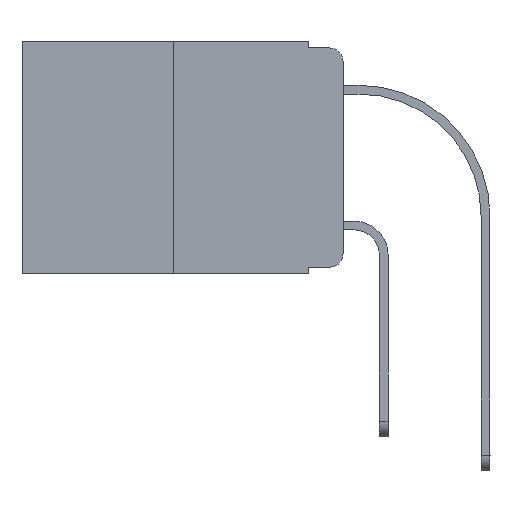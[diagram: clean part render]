
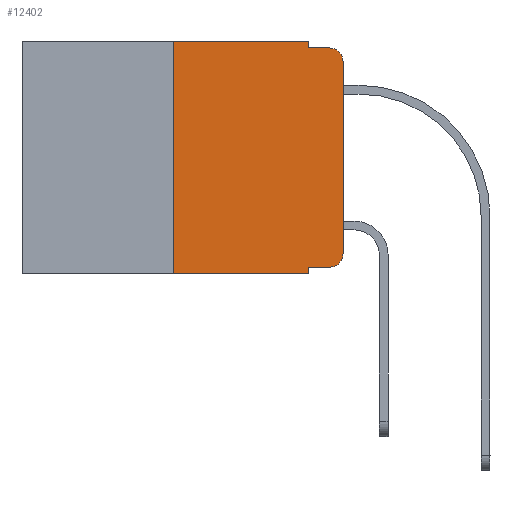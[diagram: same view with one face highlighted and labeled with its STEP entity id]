
A CAD part, left-side view. The second image highlights one B-rep face of the part: STEP entity #12402.
In plain terms, the highlighted planar face has unit normal (-1, 0, 0).
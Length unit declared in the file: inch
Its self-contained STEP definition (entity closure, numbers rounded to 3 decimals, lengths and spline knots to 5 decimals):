
#48 = CARTESIAN_POINT ( 'NONE',  ( 0., 0., -0.03 ) ) ;
#959 = CARTESIAN_POINT ( 'NONE',  ( 0., 0., 0. ) ) ;
#1026 = EDGE_CURVE ( 'NONE', #12357, #7977, #12486, .T. ) ;
#1219 = CARTESIAN_POINT ( 'NONE',  ( 0., 0.473, 0. ) ) ;
#1285 = ORIENTED_EDGE ( 'NONE', *, *, #20012, .F. ) ;
#1403 = DIRECTION ( 'NONE',  ( 0., -1., 0. ) ) ;
#2087 = CARTESIAN_POINT ( 'NONE',  ( 0., 0.051, 0. ) ) ;
#2621 = CARTESIAN_POINT ( 'NONE',  ( 0., 0.051, 0. ) ) ;
#2697 = ORIENTED_EDGE ( 'NONE', *, *, #5243, .F. ) ;
#3816 = ORIENTED_EDGE ( 'NONE', *, *, #8932, .T. ) ;
#4022 = DIRECTION ( 'NONE',  ( -1., 0., 0. ) ) ;
#4285 = CARTESIAN_POINT ( 'NONE',  ( 0., 0.051, -0.01 ) ) ;
#4560 = VERTEX_POINT ( 'NONE', #48 ) ;
#4965 = CIRCLE ( 'NONE', #16002, 0.02 ) ;
#5157 = EDGE_CURVE ( 'NONE', #23878, #4560, #9009, .T. ) ;
#5243 = EDGE_CURVE ( 'NONE', #7963, #17933, #9674, .T. ) ;
#5247 = DIRECTION ( 'NONE',  ( 0., 0., 1. ) ) ;
#5505 = EDGE_LOOP ( 'NONE', ( #9695, #7237, #6449, #23156, #2697, #14933, #5924, #1285, #17337, #3816 ) ) ;
#5670 = AXIS2_PLACEMENT_3D ( 'NONE', #8058, #4022, #8195 ) ;
#5687 = VECTOR ( 'NONE', #26960, 39.37008 ) ;
#5924 = ORIENTED_EDGE ( 'NONE', *, *, #17755, .T. ) ;
#6449 = ORIENTED_EDGE ( 'NONE', *, *, #12979, .F. ) ;
#7237 = ORIENTED_EDGE ( 'NONE', *, *, #14172, .T. ) ;
#7654 = VECTOR ( 'NONE', #1403, 39.37008 ) ;
#7759 = CARTESIAN_POINT ( 'NONE',  ( 0., 0.051, -0.343 ) ) ;
#7963 = VERTEX_POINT ( 'NONE', #9833 ) ;
#7977 = VERTEX_POINT ( 'NONE', #13708 ) ;
#8058 = CARTESIAN_POINT ( 'NONE',  ( 0., 0.02, -0.03 ) ) ;
#8102 = DIRECTION ( 'NONE',  ( 0., 0., -1. ) ) ;
#8195 = DIRECTION ( 'NONE',  ( 0., 0., -1. ) ) ;
#8223 = CARTESIAN_POINT ( 'NONE',  ( 0., 0.473, 0. ) ) ;
#8375 = VECTOR ( 'NONE', #5247, 39.37008 ) ;
#8598 = DIRECTION ( 'NONE',  ( 0., -1., 0. ) ) ;
#8600 = CARTESIAN_POINT ( 'NONE',  ( 0., 0., -0.313 ) ) ;
#8932 = EDGE_CURVE ( 'NONE', #7977, #23878, #4965, .T. ) ;
#9005 = LINE ( 'NONE', #2621, #13215 ) ;
#9009 = LINE ( 'NONE', #959, #8375 ) ;
#9391 = LINE ( 'NONE', #17819, #15899 ) ;
#9532 = VECTOR ( 'NONE', #11385, 39.37008 ) ;
#9674 = LINE ( 'NONE', #1219, #5687 ) ;
#9695 = ORIENTED_EDGE ( 'NONE', *, *, #5157, .T. ) ;
#9833 = CARTESIAN_POINT ( 'NONE',  ( 0., 0.25, 0. ) ) ;
#10539 = DIRECTION ( 'NONE',  ( 0., 0., -1. ) ) ;
#11280 = CARTESIAN_POINT ( 'NONE',  ( 0., 0.051, -0.01 ) ) ;
#11385 = DIRECTION ( 'NONE',  ( 0., -1., 0. ) ) ;
#12126 = VERTEX_POINT ( 'NONE', #11280 ) ;
#12357 = VERTEX_POINT ( 'NONE', #17770 ) ;
#12402 = ADVANCED_FACE ( 'NONE', ( #16648 ), #18984, .F. ) ;
#12486 = LINE ( 'NONE', #16341, #7654 ) ;
#12683 = AXIS2_PLACEMENT_3D ( 'NONE', #8223, #25209, #22854 ) ;
#12898 = VECTOR ( 'NONE', #18424, 39.37008 ) ;
#12979 = EDGE_CURVE ( 'NONE', #12126, #16287, #25316, .T. ) ;
#13075 = EDGE_CURVE ( 'NONE', #17933, #12126, #9005, .T. ) ;
#13215 = VECTOR ( 'NONE', #10539, 39.37008 ) ;
#13598 = LINE ( 'NONE', #21877, #9532 ) ;
#13644 = VECTOR ( 'NONE', #8598, 39.37008 ) ;
#13708 = CARTESIAN_POINT ( 'NONE',  ( 0., 0.02, -0.333 ) ) ;
#14072 = DIRECTION ( 'NONE',  ( 0., 0., -1. ) ) ;
#14172 = EDGE_CURVE ( 'NONE', #4560, #16287, #16282, .T. ) ;
#14933 = ORIENTED_EDGE ( 'NONE', *, *, #22065, .F. ) ;
#15899 = VECTOR ( 'NONE', #14072, 39.37008 ) ;
#16002 = AXIS2_PLACEMENT_3D ( 'NONE', #22739, #27052, #8102 ) ;
#16282 = CIRCLE ( 'NONE', #5670, 0.02 ) ;
#16287 = VERTEX_POINT ( 'NONE', #18842 ) ;
#16341 = CARTESIAN_POINT ( 'NONE',  ( 0., 0.051, -0.333 ) ) ;
#16648 = FACE_OUTER_BOUND ( 'NONE', #5505, .T. ) ;
#17337 = ORIENTED_EDGE ( 'NONE', *, *, #1026, .T. ) ;
#17755 = EDGE_CURVE ( 'NONE', #26178, #24984, #13598, .T. ) ;
#17770 = CARTESIAN_POINT ( 'NONE',  ( 0., 0.051, -0.333 ) ) ;
#17819 = CARTESIAN_POINT ( 'NONE',  ( 0., 0.051, 0. ) ) ;
#17933 = VERTEX_POINT ( 'NONE', #2087 ) ;
#18391 = CARTESIAN_POINT ( 'NONE',  ( 0., 0.25, -0.343 ) ) ;
#18424 = DIRECTION ( 'NONE',  ( 0., 0., 1. ) ) ;
#18842 = CARTESIAN_POINT ( 'NONE',  ( 0., 0.02, -0.01 ) ) ;
#18984 = PLANE ( 'NONE',  #12683 ) ;
#20012 = EDGE_CURVE ( 'NONE', #12357, #24984, #9391, .T. ) ;
#21877 = CARTESIAN_POINT ( 'NONE',  ( 0., 0.473, -0.343 ) ) ;
#22065 = EDGE_CURVE ( 'NONE', #26178, #7963, #24926, .T. ) ;
#22570 = CARTESIAN_POINT ( 'NONE',  ( 0., 0.25, 0. ) ) ;
#22739 = CARTESIAN_POINT ( 'NONE',  ( 0., 0.02, -0.313 ) ) ;
#22854 = DIRECTION ( 'NONE',  ( 0., 0., -1. ) ) ;
#23156 = ORIENTED_EDGE ( 'NONE', *, *, #13075, .F. ) ;
#23878 = VERTEX_POINT ( 'NONE', #8600 ) ;
#24926 = LINE ( 'NONE', #22570, #12898 ) ;
#24984 = VERTEX_POINT ( 'NONE', #7759 ) ;
#25209 = DIRECTION ( 'NONE',  ( 1., 0., 0. ) ) ;
#25316 = LINE ( 'NONE', #4285, #13644 ) ;
#26178 = VERTEX_POINT ( 'NONE', #18391 ) ;
#26960 = DIRECTION ( 'NONE',  ( 0., -1., 0. ) ) ;
#27052 = DIRECTION ( 'NONE',  ( -1., 0., 0. ) ) ;
